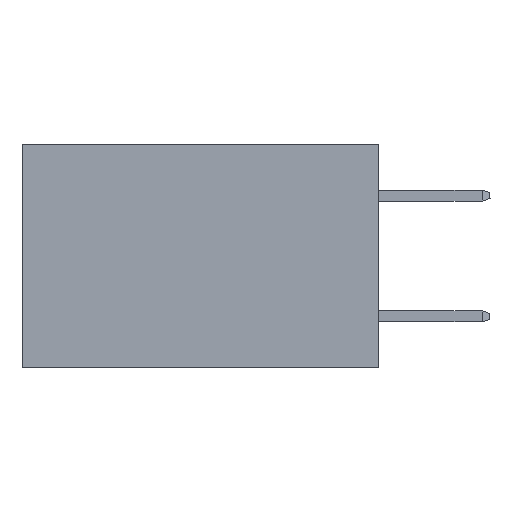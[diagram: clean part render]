
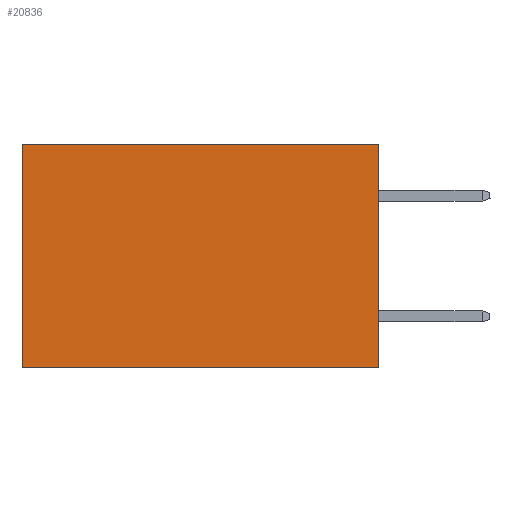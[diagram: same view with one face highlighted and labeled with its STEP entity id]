
A CAD part, left-side view. The second image highlights one B-rep face of the part: STEP entity #20836.
In plain terms, the highlighted planar face has unit normal (-1, 0, 0).
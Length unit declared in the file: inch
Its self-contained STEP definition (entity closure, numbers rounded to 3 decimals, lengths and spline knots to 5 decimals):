
#452 = ORIENTED_EDGE ( 'NONE', *, *, #3443, .T. ) ;
#559 = ORIENTED_EDGE ( 'NONE', *, *, #4297, .F. ) ;
#638 = VECTOR ( 'NONE', #8849, 39.37008 ) ;
#1974 = CARTESIAN_POINT ( 'NONE',  ( 0.277, 0., -0.37 ) ) ;
#2007 = DIRECTION ( 'NONE',  ( 0., 0., -1. ) ) ;
#2573 = VECTOR ( 'NONE', #2007, 39.37008 ) ;
#3028 = EDGE_CURVE ( 'NONE', #21139, #15109, #18029, .T. ) ;
#3443 = EDGE_CURVE ( 'NONE', #21139, #17518, #17999, .T. ) ;
#3630 = LINE ( 'NONE', #15939, #18988 ) ;
#4297 = EDGE_CURVE ( 'NONE', #15109, #22235, #3630, .T. ) ;
#5985 = CARTESIAN_POINT ( 'NONE',  ( 0.277, 0.59, -0.37 ) ) ;
#7158 = FACE_OUTER_BOUND ( 'NONE', #22491, .T. ) ;
#8331 = DIRECTION ( 'NONE',  ( 0., 0., -1. ) ) ;
#8828 = LINE ( 'NONE', #12415, #2573 ) ;
#8849 = DIRECTION ( 'NONE',  ( 0., 0., -1. ) ) ;
#11607 = CARTESIAN_POINT ( 'NONE',  ( 0.277, 0.59, 0. ) ) ;
#12355 = ORIENTED_EDGE ( 'NONE', *, *, #3028, .F. ) ;
#12393 = VECTOR ( 'NONE', #20716, 39.37008 ) ;
#12415 = CARTESIAN_POINT ( 'NONE',  ( 0.277, 0.59, -0.37 ) ) ;
#15109 = VERTEX_POINT ( 'NONE', #18806 ) ;
#15285 = DIRECTION ( 'NONE',  ( 0., 1., 0. ) ) ;
#15939 = CARTESIAN_POINT ( 'NONE',  ( 0.277, 0., -0.37 ) ) ;
#16897 = ORIENTED_EDGE ( 'NONE', *, *, #20094, .T. ) ;
#17518 = VERTEX_POINT ( 'NONE', #11607 ) ;
#17999 = LINE ( 'NONE', #24411, #12393 ) ;
#18029 = LINE ( 'NONE', #22464, #638 ) ;
#18655 = PLANE ( 'NONE',  #24307 ) ;
#18806 = CARTESIAN_POINT ( 'NONE',  ( 0.277, 0., -0.37 ) ) ;
#18988 = VECTOR ( 'NONE', #15285, 39.37008 ) ;
#20094 = EDGE_CURVE ( 'NONE', #17518, #22235, #8828, .T. ) ;
#20716 = DIRECTION ( 'NONE',  ( 0., 1., 0. ) ) ;
#20836 = ADVANCED_FACE ( 'NONE', ( #7158 ), #18655, .F. ) ;
#20912 = DIRECTION ( 'NONE',  ( 1., 0., 0. ) ) ;
#21139 = VERTEX_POINT ( 'NONE', #23963 ) ;
#22235 = VERTEX_POINT ( 'NONE', #5985 ) ;
#22464 = CARTESIAN_POINT ( 'NONE',  ( 0.277, 0., -0.37 ) ) ;
#22491 = EDGE_LOOP ( 'NONE', ( #16897, #559, #12355, #452 ) ) ;
#23963 = CARTESIAN_POINT ( 'NONE',  ( 0.277, 0., 0. ) ) ;
#24307 = AXIS2_PLACEMENT_3D ( 'NONE', #1974, #20912, #8331 ) ;
#24411 = CARTESIAN_POINT ( 'NONE',  ( 0.277, 0., 0. ) ) ;
